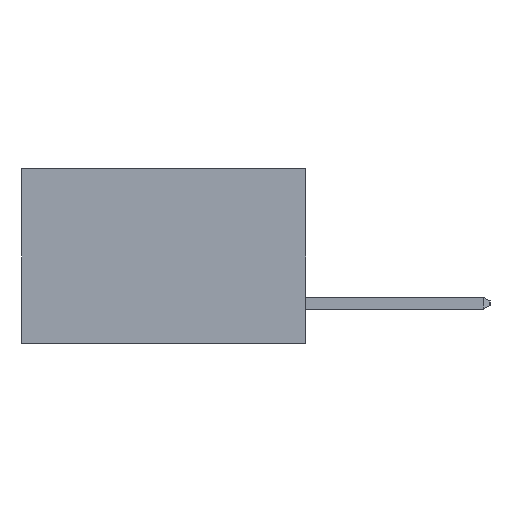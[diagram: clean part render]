
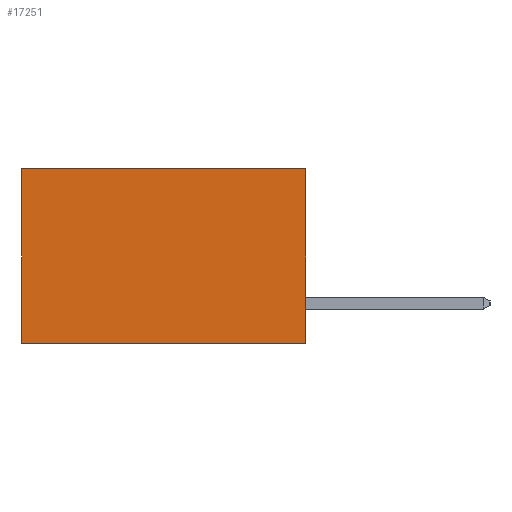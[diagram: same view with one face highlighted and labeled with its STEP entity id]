
A CAD part, left-side view. The second image highlights one B-rep face of the part: STEP entity #17251.
In plain terms, the highlighted planar face has unit normal (-1, 0, 0).
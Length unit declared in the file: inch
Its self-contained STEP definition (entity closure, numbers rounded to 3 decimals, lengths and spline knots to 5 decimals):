
#1689 = DIRECTION ( 'NONE',  ( 0., 0., -1. ) ) ;
#2046 = FACE_OUTER_BOUND ( 'NONE', #16695, .T. ) ;
#2195 = LINE ( 'NONE', #2509, #19392 ) ;
#2457 = VERTEX_POINT ( 'NONE', #18187 ) ;
#2509 = CARTESIAN_POINT ( 'NONE',  ( 0.2615, 0., -0.37 ) ) ;
#4309 = AXIS2_PLACEMENT_3D ( 'NONE', #21412, #11817, #1689 ) ;
#4828 = LINE ( 'NONE', #18713, #18007 ) ;
#6513 = VECTOR ( 'NONE', #11412, 39.37008 ) ;
#7103 = EDGE_CURVE ( 'NONE', #12614, #10322, #11065, .T. ) ;
#10322 = VERTEX_POINT ( 'NONE', #20770 ) ;
#10831 = ORIENTED_EDGE ( 'NONE', *, *, #7103, .T. ) ;
#11006 = DIRECTION ( 'NONE',  ( 0., 0., -1. ) ) ;
#11065 = LINE ( 'NONE', #19236, #16022 ) ;
#11349 = CARTESIAN_POINT ( 'NONE',  ( 0.2615, 0., 0. ) ) ;
#11412 = DIRECTION ( 'NONE',  ( 0., 1., 0. ) ) ;
#11737 = CARTESIAN_POINT ( 'NONE',  ( 0.2615, 0.6, 0. ) ) ;
#11817 = DIRECTION ( 'NONE',  ( 1., 0., 0. ) ) ;
#12424 = EDGE_CURVE ( 'NONE', #19182, #10322, #4828, .T. ) ;
#12606 = ORIENTED_EDGE ( 'NONE', *, *, #20054, .F. ) ;
#12614 = VERTEX_POINT ( 'NONE', #11737 ) ;
#14349 = ORIENTED_EDGE ( 'NONE', *, *, #12424, .F. ) ;
#16022 = VECTOR ( 'NONE', #19118, 39.37008 ) ;
#16695 = EDGE_LOOP ( 'NONE', ( #10831, #14349, #12606, #18834 ) ) ;
#17251 = ADVANCED_FACE ( 'NONE', ( #2046 ), #21470, .F. ) ;
#18007 = VECTOR ( 'NONE', #18663, 39.37008 ) ;
#18187 = CARTESIAN_POINT ( 'NONE',  ( 0.2615, 0., 0. ) ) ;
#18663 = DIRECTION ( 'NONE',  ( 0., 1., 0. ) ) ;
#18713 = CARTESIAN_POINT ( 'NONE',  ( 0.2615, 0., -0.37 ) ) ;
#18834 = ORIENTED_EDGE ( 'NONE', *, *, #20680, .T. ) ;
#19108 = LINE ( 'NONE', #11349, #6513 ) ;
#19118 = DIRECTION ( 'NONE',  ( 0., 0., -1. ) ) ;
#19182 = VERTEX_POINT ( 'NONE', #20236 ) ;
#19236 = CARTESIAN_POINT ( 'NONE',  ( 0.2615, 0.6, -0.37 ) ) ;
#19392 = VECTOR ( 'NONE', #11006, 39.37008 ) ;
#20054 = EDGE_CURVE ( 'NONE', #2457, #19182, #2195, .T. ) ;
#20236 = CARTESIAN_POINT ( 'NONE',  ( 0.2615, 0., -0.37 ) ) ;
#20680 = EDGE_CURVE ( 'NONE', #2457, #12614, #19108, .T. ) ;
#20770 = CARTESIAN_POINT ( 'NONE',  ( 0.2615, 0.6, -0.37 ) ) ;
#21412 = CARTESIAN_POINT ( 'NONE',  ( 0.2615, 0., -0.37 ) ) ;
#21470 = PLANE ( 'NONE',  #4309 ) ;
